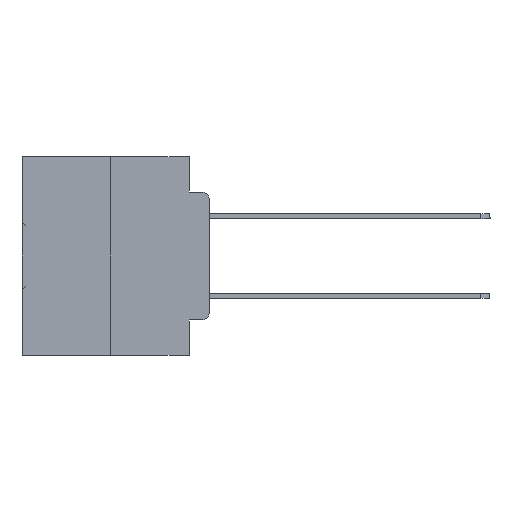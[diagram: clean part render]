
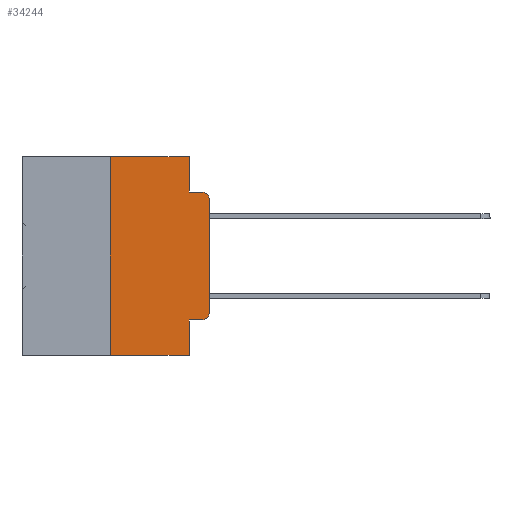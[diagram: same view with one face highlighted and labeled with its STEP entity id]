
A CAD part, left-side view. The second image highlights one B-rep face of the part: STEP entity #34244.
In plain terms, the highlighted planar face has unit normal (-1, 0, 0).
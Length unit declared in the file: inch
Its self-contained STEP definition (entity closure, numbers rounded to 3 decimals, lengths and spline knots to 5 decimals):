
#159 = CARTESIAN_POINT ( 'NONE',  ( 0., 0.051, -0.0885 ) ) ;
#258 = EDGE_CURVE ( 'NONE', #19911, #3742, #31608, .T. ) ;
#774 = DIRECTION ( 'NONE',  ( -1., 0., 0. ) ) ;
#958 = DIRECTION ( 'NONE',  ( 0., 0., -1. ) ) ;
#1113 = CARTESIAN_POINT ( 'NONE',  ( 0., 0.051, -0.5 ) ) ;
#1214 = ORIENTED_EDGE ( 'NONE', *, *, #19256, .T. ) ;
#1743 = DIRECTION ( 'NONE',  ( 1., 0., 0. ) ) ;
#2958 = DIRECTION ( 'NONE',  ( 0., -1., 0. ) ) ;
#3742 = VERTEX_POINT ( 'NONE', #159 ) ;
#4231 = LINE ( 'NONE', #31109, #8329 ) ;
#4240 = ORIENTED_EDGE ( 'NONE', *, *, #17337, .F. ) ;
#4347 = VERTEX_POINT ( 'NONE', #35436 ) ;
#4433 = CARTESIAN_POINT ( 'NONE',  ( 0., 0.25, 0. ) ) ;
#4466 = CARTESIAN_POINT ( 'NONE',  ( 0., 0.473, -0.5 ) ) ;
#4707 = AXIS2_PLACEMENT_3D ( 'NONE', #15237, #774, #29963 ) ;
#5710 = DIRECTION ( 'NONE',  ( 0., -1., 0. ) ) ;
#6599 = EDGE_CURVE ( 'NONE', #21793, #11849, #4231, .T. ) ;
#6820 = CARTESIAN_POINT ( 'NONE',  ( 0., 0.051, -0.0885 ) ) ;
#7086 = VERTEX_POINT ( 'NONE', #1113 ) ;
#8318 = EDGE_CURVE ( 'NONE', #10735, #32526, #17297, .T. ) ;
#8329 = VECTOR ( 'NONE', #13696, 39.37008 ) ;
#8339 = CARTESIAN_POINT ( 'NONE',  ( 0., 0.25, -0.5 ) ) ;
#8617 = FACE_OUTER_BOUND ( 'NONE', #27175, .T. ) ;
#9353 = CARTESIAN_POINT ( 'NONE',  ( 0., 0.051, 0. ) ) ;
#9606 = CARTESIAN_POINT ( 'NONE',  ( 0., 0.02, -0.4115 ) ) ;
#9863 = DIRECTION ( 'NONE',  ( 0., -1., 0. ) ) ;
#10004 = ORIENTED_EDGE ( 'NONE', *, *, #27457, .T. ) ;
#10135 = CARTESIAN_POINT ( 'NONE',  ( 0., 0.02, -0.3915 ) ) ;
#10644 = VECTOR ( 'NONE', #9863, 39.37008 ) ;
#10735 = VERTEX_POINT ( 'NONE', #8339 ) ;
#11407 = EDGE_CURVE ( 'NONE', #4347, #16781, #33353, .T. ) ;
#11684 = DIRECTION ( 'NONE',  ( 0., 0., -1. ) ) ;
#11849 = VERTEX_POINT ( 'NONE', #19452 ) ;
#11921 = CARTESIAN_POINT ( 'NONE',  ( 0., 0.473, 0. ) ) ;
#12751 = EDGE_CURVE ( 'NONE', #4347, #7086, #31864, .T. ) ;
#12866 = VECTOR ( 'NONE', #30641, 39.37008 ) ;
#13696 = DIRECTION ( 'NONE',  ( 0., 0., 1. ) ) ;
#13977 = VERTEX_POINT ( 'NONE', #37649 ) ;
#14091 = ORIENTED_EDGE ( 'NONE', *, *, #8318, .F. ) ;
#14183 = LINE ( 'NONE', #11921, #19219 ) ;
#14464 = VECTOR ( 'NONE', #958, 39.37008 ) ;
#14757 = LINE ( 'NONE', #6820, #10644 ) ;
#14823 = CARTESIAN_POINT ( 'NONE',  ( 0., 0.051, 0. ) ) ;
#15237 = CARTESIAN_POINT ( 'NONE',  ( 0., 0.02, -0.1085 ) ) ;
#15367 = ORIENTED_EDGE ( 'NONE', *, *, #258, .F. ) ;
#16376 = AXIS2_PLACEMENT_3D ( 'NONE', #28035, #1743, #36898 ) ;
#16781 = VERTEX_POINT ( 'NONE', #9606 ) ;
#17297 = LINE ( 'NONE', #24199, #27867 ) ;
#17337 = EDGE_CURVE ( 'NONE', #32526, #19911, #14183, .T. ) ;
#18863 = ORIENTED_EDGE ( 'NONE', *, *, #6599, .T. ) ;
#19219 = VECTOR ( 'NONE', #5710, 39.37008 ) ;
#19256 = EDGE_CURVE ( 'NONE', #11849, #13977, #21335, .T. ) ;
#19452 = CARTESIAN_POINT ( 'NONE',  ( 0., 0., -0.1085 ) ) ;
#19615 = ORIENTED_EDGE ( 'NONE', *, *, #34007, .T. ) ;
#19911 = VERTEX_POINT ( 'NONE', #14823 ) ;
#21238 = DIRECTION ( 'NONE',  ( 0., 0., 1. ) ) ;
#21335 = CIRCLE ( 'NONE', #4707, 0.02 ) ;
#21793 = VERTEX_POINT ( 'NONE', #24227 ) ;
#21908 = VECTOR ( 'NONE', #2958, 39.37008 ) ;
#22904 = VECTOR ( 'NONE', #11684, 39.37008 ) ;
#24199 = CARTESIAN_POINT ( 'NONE',  ( 0., 0.25, 0. ) ) ;
#24227 = CARTESIAN_POINT ( 'NONE',  ( 0., 0., -0.3915 ) ) ;
#27175 = EDGE_LOOP ( 'NONE', ( #18863, #1214, #34528, #15367, #4240, #14091, #10004, #35007, #37628, #19615 ) ) ;
#27441 = CARTESIAN_POINT ( 'NONE',  ( 0., 0.051, 0. ) ) ;
#27457 = EDGE_CURVE ( 'NONE', #10735, #7086, #28899, .T. ) ;
#27867 = VECTOR ( 'NONE', #21238, 39.37008 ) ;
#28035 = CARTESIAN_POINT ( 'NONE',  ( 0., 0.473, 0. ) ) ;
#28899 = LINE ( 'NONE', #4466, #12866 ) ;
#29963 = DIRECTION ( 'NONE',  ( 0., 0., -1. ) ) ;
#30641 = DIRECTION ( 'NONE',  ( 0., -1., 0. ) ) ;
#31109 = CARTESIAN_POINT ( 'NONE',  ( 0., 0., 0. ) ) ;
#31608 = LINE ( 'NONE', #27441, #22904 ) ;
#31864 = LINE ( 'NONE', #9353, #14464 ) ;
#32160 = CARTESIAN_POINT ( 'NONE',  ( 0., 0.051, -0.4115 ) ) ;
#32328 = AXIS2_PLACEMENT_3D ( 'NONE', #10135, #35778, #36029 ) ;
#32526 = VERTEX_POINT ( 'NONE', #4433 ) ;
#33353 = LINE ( 'NONE', #32160, #21908 ) ;
#34007 = EDGE_CURVE ( 'NONE', #16781, #21793, #35581, .T. ) ;
#34244 = ADVANCED_FACE ( 'NONE', ( #8617 ), #36775, .F. ) ;
#34528 = ORIENTED_EDGE ( 'NONE', *, *, #37248, .F. ) ;
#35007 = ORIENTED_EDGE ( 'NONE', *, *, #12751, .F. ) ;
#35436 = CARTESIAN_POINT ( 'NONE',  ( 0., 0.051, -0.4115 ) ) ;
#35581 = CIRCLE ( 'NONE', #32328, 0.02 ) ;
#35778 = DIRECTION ( 'NONE',  ( -1., 0., 0. ) ) ;
#36029 = DIRECTION ( 'NONE',  ( 0., 0., -1. ) ) ;
#36775 = PLANE ( 'NONE',  #16376 ) ;
#36898 = DIRECTION ( 'NONE',  ( 0., 0., -1. ) ) ;
#37248 = EDGE_CURVE ( 'NONE', #3742, #13977, #14757, .T. ) ;
#37628 = ORIENTED_EDGE ( 'NONE', *, *, #11407, .T. ) ;
#37649 = CARTESIAN_POINT ( 'NONE',  ( 0., 0.02, -0.0885 ) ) ;
